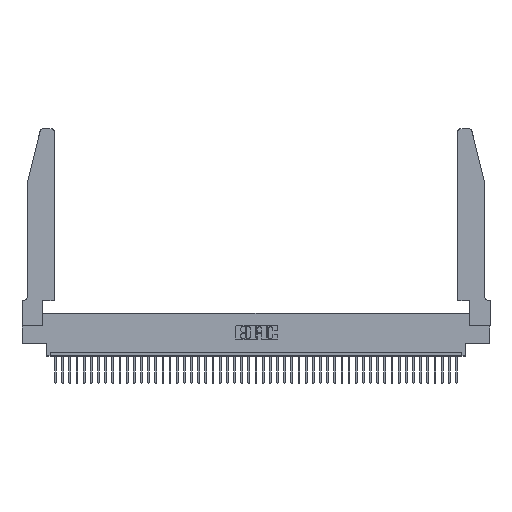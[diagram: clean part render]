
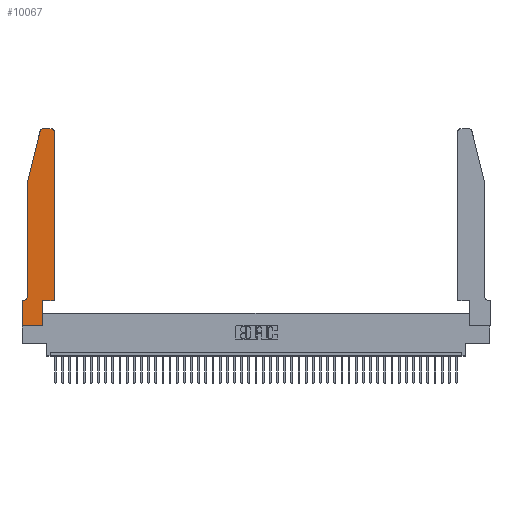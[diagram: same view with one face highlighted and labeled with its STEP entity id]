
A CAD part, top view. The second image highlights one B-rep face of the part: STEP entity #10067.
In plain terms, the highlighted planar face has unit normal (0, 0, 1).
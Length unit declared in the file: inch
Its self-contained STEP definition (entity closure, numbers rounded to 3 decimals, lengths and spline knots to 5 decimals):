
#212 = EDGE_CURVE ( 'NONE', #44404, #25379, #27682, .T. ) ;
#341 = DIRECTION ( 'NONE',  ( 1., 0., 0. ) ) ;
#926 = ORIENTED_EDGE ( 'NONE', *, *, #10744, .T. ) ;
#1179 = ORIENTED_EDGE ( 'NONE', *, *, #5879, .T. ) ;
#1428 = EDGE_CURVE ( 'NONE', #21774, #4756, #13148, .T. ) ;
#1456 = CARTESIAN_POINT ( 'NONE',  ( 0.2865, 0.35, 0.37 ) ) ;
#1957 = LINE ( 'NONE', #27083, #45632 ) ;
#2771 = VERTEX_POINT ( 'NONE', #23827 ) ;
#3070 = CARTESIAN_POINT ( 'NONE',  ( 0., 0.35, 0.37 ) ) ;
#3219 = PLANE ( 'NONE',  #33498 ) ;
#3227 = DIRECTION ( 'NONE',  ( 1., 0., 0. ) ) ;
#4756 = VERTEX_POINT ( 'NONE', #42892 ) ;
#4846 = ORIENTED_EDGE ( 'NONE', *, *, #212, .T. ) ;
#5879 = EDGE_CURVE ( 'NONE', #24024, #21774, #20152, .T. ) ;
#6045 = VERTEX_POINT ( 'NONE', #36410 ) ;
#6201 = DIRECTION ( 'NONE',  ( 0., -1., 0. ) ) ;
#6382 = ORIENTED_EDGE ( 'NONE', *, *, #12207, .T. ) ;
#7218 = DIRECTION ( 'NONE',  ( -1., 0., 0. ) ) ;
#7626 = AXIS2_PLACEMENT_3D ( 'NONE', #42814, #18285, #341 ) ;
#7795 = CIRCLE ( 'NONE', #39082, 0.03 ) ;
#8248 = CARTESIAN_POINT ( 'NONE',  ( 0.4505, 0.35, 0.37 ) ) ;
#8609 = DIRECTION ( 'NONE',  ( 0., -1., 0. ) ) ;
#9338 = VECTOR ( 'NONE', #40432, 39.37008 ) ;
#9537 = VECTOR ( 'NONE', #25541, 39.37008 ) ;
#9553 = ORIENTED_EDGE ( 'NONE', *, *, #17939, .T. ) ;
#9952 = CARTESIAN_POINT ( 'NONE',  ( 0.2865, 0., 0.37 ) ) ;
#10067 = ADVANCED_FACE ( 'NONE', ( #34101 ), #3219, .T. ) ;
#10327 = CARTESIAN_POINT ( 'NONE',  ( 0.4505, 2.72, 0.37 ) ) ;
#10744 = EDGE_CURVE ( 'NONE', #44932, #34188, #1957, .T. ) ;
#11744 = CARTESIAN_POINT ( 'NONE',  ( 0.0055, 0.42, 0.37 ) ) ;
#11894 = DIRECTION ( 'NONE',  ( 0., 0., -1. ) ) ;
#12207 = EDGE_CURVE ( 'NONE', #2771, #24024, #29286, .T. ) ;
#12619 = EDGE_CURVE ( 'NONE', #34188, #30311, #27620, .T. ) ;
#13148 = CIRCLE ( 'NONE', #20954, 0.07 ) ;
#13736 = CARTESIAN_POINT ( 'NONE',  ( 0.284, 2.72, 0.37 ) ) ;
#13738 = CARTESIAN_POINT ( 'NONE',  ( 0.0755, 0.35, 0.37 ) ) ;
#17079 = EDGE_CURVE ( 'NONE', #6045, #44932, #18933, .T. ) ;
#17939 = EDGE_CURVE ( 'NONE', #25379, #33578, #34508, .T. ) ;
#18285 = DIRECTION ( 'NONE',  ( 0., 0., 1. ) ) ;
#18368 = CARTESIAN_POINT ( 'NONE',  ( 0., 0.35, 0.37 ) ) ;
#18582 = VECTOR ( 'NONE', #22450, 39.37008 ) ;
#18933 = LINE ( 'NONE', #38332, #9537 ) ;
#19201 = CARTESIAN_POINT ( 'NONE',  ( 0., 0., 0.37 ) ) ;
#19347 = CARTESIAN_POINT ( 'NONE',  ( 0.4205, 2.75, 0.37 ) ) ;
#19707 = VERTEX_POINT ( 'NONE', #18368 ) ;
#20152 = LINE ( 'NONE', #43328, #37772 ) ;
#20236 = DIRECTION ( 'NONE',  ( 1., 0., 0. ) ) ;
#20257 = EDGE_CURVE ( 'NONE', #33578, #2771, #7795, .T. ) ;
#20869 = CARTESIAN_POINT ( 'NONE',  ( 0.284, 2.75, 0.37 ) ) ;
#20954 = AXIS2_PLACEMENT_3D ( 'NONE', #11744, #11894, #25642 ) ;
#21774 = VERTEX_POINT ( 'NONE', #23665 ) ;
#22450 = DIRECTION ( 'NONE',  ( 0., 1., 0. ) ) ;
#22457 = LINE ( 'NONE', #8248, #18582 ) ;
#22834 = EDGE_CURVE ( 'NONE', #19707, #6045, #23583, .T. ) ;
#23583 = LINE ( 'NONE', #19201, #39572 ) ;
#23665 = CARTESIAN_POINT ( 'NONE',  ( 0.0755, 0.42, 0.37 ) ) ;
#23827 = CARTESIAN_POINT ( 'NONE',  ( 0.25487, 2.72718, 0.37 ) ) ;
#23885 = EDGE_CURVE ( 'NONE', #30311, #44404, #22457, .T. ) ;
#23984 = DIRECTION ( 'NONE',  ( 0., 1., 0. ) ) ;
#24024 = VERTEX_POINT ( 'NONE', #25657 ) ;
#24654 = DIRECTION ( 'NONE',  ( -0.239, -0.971, 0. ) ) ;
#25379 = VERTEX_POINT ( 'NONE', #19347 ) ;
#25541 = DIRECTION ( 'NONE',  ( 1., 0., 0. ) ) ;
#25642 = DIRECTION ( 'NONE',  ( -1., 0., 0. ) ) ;
#25657 = CARTESIAN_POINT ( 'NONE',  ( 0.0755, 2., 0.37 ) ) ;
#26822 = CARTESIAN_POINT ( 'NONE',  ( 0.4505, 0.35, 0.37 ) ) ;
#26921 = EDGE_CURVE ( 'NONE', #4756, #19707, #28313, .T. ) ;
#27083 = CARTESIAN_POINT ( 'NONE',  ( 0.2865, 0.35, 0.37 ) ) ;
#27620 = LINE ( 'NONE', #33193, #9338 ) ;
#27682 = CIRCLE ( 'NONE', #7626, 0.03 ) ;
#27819 = DIRECTION ( 'NONE',  ( 0., 0., 1. ) ) ;
#28313 = LINE ( 'NONE', #13738, #31032 ) ;
#28331 = CARTESIAN_POINT ( 'NONE',  ( 0.0755, 2., 0.37 ) ) ;
#29286 = LINE ( 'NONE', #28331, #32010 ) ;
#29781 = EDGE_LOOP ( 'NONE', ( #9553, #39781, #6382, #1179, #40528, #31661, #44736, #35427, #926, #41049, #40006, #4846 ) ) ;
#30311 = VERTEX_POINT ( 'NONE', #26822 ) ;
#31032 = VECTOR ( 'NONE', #38430, 39.37008 ) ;
#31661 = ORIENTED_EDGE ( 'NONE', *, *, #26921, .T. ) ;
#31793 = DIRECTION ( 'NONE',  ( 0., 0., 1. ) ) ;
#32010 = VECTOR ( 'NONE', #24654, 39.37008 ) ;
#33193 = CARTESIAN_POINT ( 'NONE',  ( 0.4505, 0.35, 0.37 ) ) ;
#33498 = AXIS2_PLACEMENT_3D ( 'NONE', #3070, #27819, #20236 ) ;
#33578 = VERTEX_POINT ( 'NONE', #20869 ) ;
#34101 = FACE_OUTER_BOUND ( 'NONE', #29781, .T. ) ;
#34188 = VERTEX_POINT ( 'NONE', #1456 ) ;
#34508 = LINE ( 'NONE', #35869, #42237 ) ;
#35427 = ORIENTED_EDGE ( 'NONE', *, *, #17079, .T. ) ;
#35869 = CARTESIAN_POINT ( 'NONE',  ( 0.2605, 2.75, 0.37 ) ) ;
#36410 = CARTESIAN_POINT ( 'NONE',  ( 0., 0., 0.37 ) ) ;
#37772 = VECTOR ( 'NONE', #8609, 39.37008 ) ;
#38332 = CARTESIAN_POINT ( 'NONE',  ( 0., 0., 0.37 ) ) ;
#38430 = DIRECTION ( 'NONE',  ( -1., 0., 0. ) ) ;
#39082 = AXIS2_PLACEMENT_3D ( 'NONE', #13736, #31793, #3227 ) ;
#39572 = VECTOR ( 'NONE', #6201, 39.37008 ) ;
#39781 = ORIENTED_EDGE ( 'NONE', *, *, #20257, .T. ) ;
#40006 = ORIENTED_EDGE ( 'NONE', *, *, #23885, .T. ) ;
#40432 = DIRECTION ( 'NONE',  ( 1., 0., 0. ) ) ;
#40528 = ORIENTED_EDGE ( 'NONE', *, *, #1428, .T. ) ;
#41049 = ORIENTED_EDGE ( 'NONE', *, *, #12619, .T. ) ;
#42237 = VECTOR ( 'NONE', #7218, 39.37008 ) ;
#42814 = CARTESIAN_POINT ( 'NONE',  ( 0.4205, 2.72, 0.37 ) ) ;
#42892 = CARTESIAN_POINT ( 'NONE',  ( 0.0055, 0.35, 0.37 ) ) ;
#43328 = CARTESIAN_POINT ( 'NONE',  ( 0.0755, 2., 0.37 ) ) ;
#44404 = VERTEX_POINT ( 'NONE', #10327 ) ;
#44736 = ORIENTED_EDGE ( 'NONE', *, *, #22834, .T. ) ;
#44932 = VERTEX_POINT ( 'NONE', #9952 ) ;
#45632 = VECTOR ( 'NONE', #23984, 39.37008 ) ;
